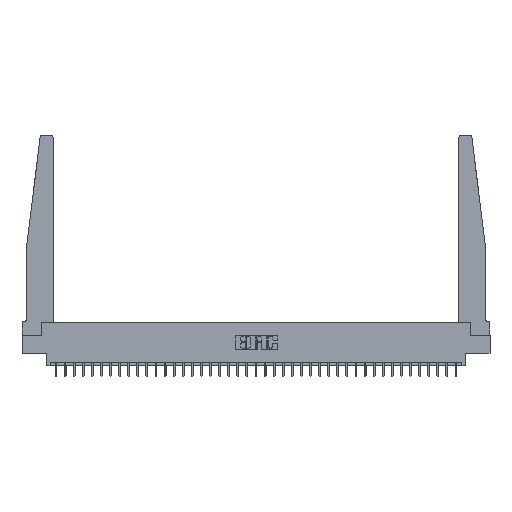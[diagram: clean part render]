
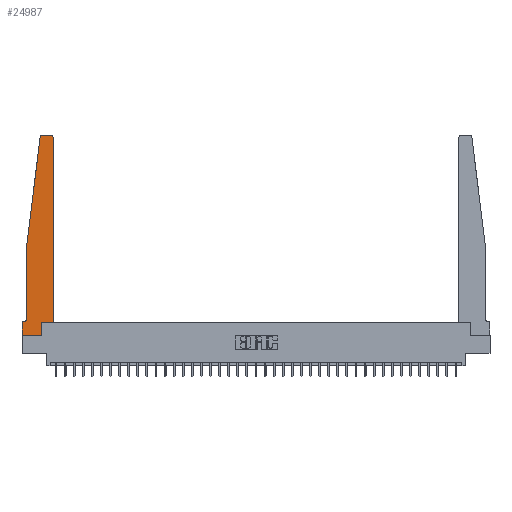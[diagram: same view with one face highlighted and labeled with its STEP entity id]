
A CAD part, top view. The second image highlights one B-rep face of the part: STEP entity #24987.
In plain terms, the highlighted planar face has unit normal (0, 0, 1).
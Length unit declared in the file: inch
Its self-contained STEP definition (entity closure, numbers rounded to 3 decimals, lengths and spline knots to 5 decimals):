
#27 = EDGE_CURVE ( 'NONE', #30497, #17124, #23463, .T. ) ;
#287 = CARTESIAN_POINT ( 'NONE',  ( 0., 0., 0.37 ) ) ;
#618 = AXIS2_PLACEMENT_3D ( 'NONE', #7165, #10270, #2116 ) ;
#1739 = DIRECTION ( 'NONE',  ( 1., 0., 0. ) ) ;
#2116 = DIRECTION ( 'NONE',  ( 1., 0., 0. ) ) ;
#2650 = VERTEX_POINT ( 'NONE', #287 ) ;
#3519 = CARTESIAN_POINT ( 'NONE',  ( 0.065, 0.1875, 0.37 ) ) ;
#5284 = VECTOR ( 'NONE', #30593, 39.37008 ) ;
#5538 = CARTESIAN_POINT ( 'NONE',  ( 0.425, 0.18, 0.37 ) ) ;
#5985 = CARTESIAN_POINT ( 'NONE',  ( 0.015, 0.1875, 0.37 ) ) ;
#6032 = CIRCLE ( 'NONE', #25410, 0.03 ) ;
#6417 = CIRCLE ( 'NONE', #11397, 0.05 ) ;
#7165 = CARTESIAN_POINT ( 'NONE',  ( 0., 0.1875, 0.37 ) ) ;
#7226 = VECTOR ( 'NONE', #32713, 39.37008 ) ;
#7527 = CARTESIAN_POINT ( 'NONE',  ( 0.2605, 0.18, 0.37 ) ) ;
#8022 = VERTEX_POINT ( 'NONE', #12897 ) ;
#8242 = AXIS2_PLACEMENT_3D ( 'NONE', #17707, #23071, #1739 ) ;
#8341 = EDGE_CURVE ( 'NONE', #2650, #33157, #9206, .T. ) ;
#8497 = VERTEX_POINT ( 'NONE', #12517 ) ;
#8962 = EDGE_CURVE ( 'NONE', #17124, #8022, #28455, .T. ) ;
#9074 = ORIENTED_EDGE ( 'NONE', *, *, #9526, .T. ) ;
#9206 = LINE ( 'NONE', #9385, #5284 ) ;
#9319 = EDGE_CURVE ( 'NONE', #31502, #16985, #12225, .T. ) ;
#9385 = CARTESIAN_POINT ( 'NONE',  ( 0., 0., 0.37 ) ) ;
#9450 = EDGE_CURVE ( 'NONE', #16985, #8497, #6032, .T. ) ;
#9526 = EDGE_CURVE ( 'NONE', #24720, #2650, #24337, .T. ) ;
#9711 = ORIENTED_EDGE ( 'NONE', *, *, #16611, .T. ) ;
#9835 = VERTEX_POINT ( 'NONE', #25703 ) ;
#10116 = CARTESIAN_POINT ( 'NONE',  ( 0.27653, 2.72, 0.37 ) ) ;
#10270 = DIRECTION ( 'NONE',  ( 0., 0., 1. ) ) ;
#11397 = AXIS2_PLACEMENT_3D ( 'NONE', #27478, #30103, #11688 ) ;
#11688 = DIRECTION ( 'NONE',  ( -1., 0., 0. ) ) ;
#12225 = LINE ( 'NONE', #22802, #24852 ) ;
#12517 = CARTESIAN_POINT ( 'NONE',  ( 0.24675, 2.72367, 0.37 ) ) ;
#12897 = CARTESIAN_POINT ( 'NONE',  ( 0.425, 2.72, 0.37 ) ) ;
#13628 = VECTOR ( 'NONE', #21528, 39.37008 ) ;
#14913 = CIRCLE ( 'NONE', #8242, 0.03 ) ;
#16009 = DIRECTION ( 'NONE',  ( 1., 0., 0. ) ) ;
#16269 = EDGE_CURVE ( 'NONE', #9835, #26635, #6417, .T. ) ;
#16300 = CARTESIAN_POINT ( 'NONE',  ( 0.065, 1.25, 0.37 ) ) ;
#16331 = LINE ( 'NONE', #21168, #13628 ) ;
#16611 = EDGE_CURVE ( 'NONE', #21790, #9835, #16331, .T. ) ;
#16985 = VERTEX_POINT ( 'NONE', #23419 ) ;
#17124 = VERTEX_POINT ( 'NONE', #5538 ) ;
#17304 = ORIENTED_EDGE ( 'NONE', *, *, #19566, .T. ) ;
#17484 = CARTESIAN_POINT ( 'NONE',  ( 0.065, 1.25, 0.37 ) ) ;
#17707 = CARTESIAN_POINT ( 'NONE',  ( 0.395, 2.72, 0.37 ) ) ;
#18349 = ORIENTED_EDGE ( 'NONE', *, *, #9319, .T. ) ;
#18661 = CARTESIAN_POINT ( 'NONE',  ( 0., 0.1875, 0.37 ) ) ;
#18758 = DIRECTION ( 'NONE',  ( 1., 0., 0. ) ) ;
#19566 = EDGE_CURVE ( 'NONE', #33157, #30497, #19835, .T. ) ;
#19835 = LINE ( 'NONE', #22263, #25959 ) ;
#20312 = EDGE_CURVE ( 'NONE', #8022, #31502, #14913, .T. ) ;
#20445 = CARTESIAN_POINT ( 'NONE',  ( 0.425, 0.18, 0.37 ) ) ;
#20695 = DIRECTION ( 'NONE',  ( 0., 0., 1. ) ) ;
#21054 = ORIENTED_EDGE ( 'NONE', *, *, #20312, .T. ) ;
#21168 = CARTESIAN_POINT ( 'NONE',  ( 0.065, 1.25, 0.37 ) ) ;
#21209 = ORIENTED_EDGE ( 'NONE', *, *, #9450, .T. ) ;
#21356 = CARTESIAN_POINT ( 'NONE',  ( 0.425, 0.18, 0.37 ) ) ;
#21528 = DIRECTION ( 'NONE',  ( 0., -1., 0. ) ) ;
#21547 = DIRECTION ( 'NONE',  ( 0., -1., 0. ) ) ;
#21790 = VERTEX_POINT ( 'NONE', #16300 ) ;
#22207 = VECTOR ( 'NONE', #28088, 39.37008 ) ;
#22263 = CARTESIAN_POINT ( 'NONE',  ( 0.2605, 0.18, 0.37 ) ) ;
#22347 = EDGE_LOOP ( 'NONE', ( #18349, #21209, #23995, #9711, #33280, #24533, #9074, #24364, #17304, #27841, #25458, #21054 ) ) ;
#22669 = VECTOR ( 'NONE', #21547, 39.37008 ) ;
#22802 = CARTESIAN_POINT ( 'NONE',  ( 0.25, 2.75, 0.37 ) ) ;
#23071 = DIRECTION ( 'NONE',  ( 0., 0., 1. ) ) ;
#23128 = DIRECTION ( 'NONE',  ( -1., 0., 0. ) ) ;
#23175 = VECTOR ( 'NONE', #23388, 39.37008 ) ;
#23294 = PLANE ( 'NONE',  #618 ) ;
#23388 = DIRECTION ( 'NONE',  ( 0., 1., 0. ) ) ;
#23419 = CARTESIAN_POINT ( 'NONE',  ( 0.27653, 2.75, 0.37 ) ) ;
#23463 = LINE ( 'NONE', #21356, #31782 ) ;
#23542 = EDGE_CURVE ( 'NONE', #26635, #24720, #27474, .T. ) ;
#23995 = ORIENTED_EDGE ( 'NONE', *, *, #30075, .T. ) ;
#24074 = CARTESIAN_POINT ( 'NONE',  ( 0.395, 2.75, 0.37 ) ) ;
#24337 = LINE ( 'NONE', #27451, #22669 ) ;
#24364 = ORIENTED_EDGE ( 'NONE', *, *, #8341, .T. ) ;
#24533 = ORIENTED_EDGE ( 'NONE', *, *, #23542, .T. ) ;
#24720 = VERTEX_POINT ( 'NONE', #18661 ) ;
#24852 = VECTOR ( 'NONE', #23128, 39.37008 ) ;
#24987 = ADVANCED_FACE ( 'NONE', ( #34242 ), #23294, .T. ) ;
#25286 = LINE ( 'NONE', #17484, #22207 ) ;
#25410 = AXIS2_PLACEMENT_3D ( 'NONE', #10116, #20695, #16009 ) ;
#25458 = ORIENTED_EDGE ( 'NONE', *, *, #8962, .T. ) ;
#25703 = CARTESIAN_POINT ( 'NONE',  ( 0.065, 0.2375, 0.37 ) ) ;
#25959 = VECTOR ( 'NONE', #30460, 39.37008 ) ;
#26635 = VERTEX_POINT ( 'NONE', #5985 ) ;
#27451 = CARTESIAN_POINT ( 'NONE',  ( 0., 0., 0.37 ) ) ;
#27474 = LINE ( 'NONE', #3519, #7226 ) ;
#27478 = CARTESIAN_POINT ( 'NONE',  ( 0.015, 0.2375, 0.37 ) ) ;
#27841 = ORIENTED_EDGE ( 'NONE', *, *, #27, .T. ) ;
#28088 = DIRECTION ( 'NONE',  ( -0.122, -0.992, 0. ) ) ;
#28455 = LINE ( 'NONE', #20445, #23175 ) ;
#28798 = CARTESIAN_POINT ( 'NONE',  ( 0.2605, 0., 0.37 ) ) ;
#30075 = EDGE_CURVE ( 'NONE', #8497, #21790, #25286, .T. ) ;
#30103 = DIRECTION ( 'NONE',  ( 0., 0., -1. ) ) ;
#30460 = DIRECTION ( 'NONE',  ( 0., 1., 0. ) ) ;
#30497 = VERTEX_POINT ( 'NONE', #7527 ) ;
#30593 = DIRECTION ( 'NONE',  ( 1., 0., 0. ) ) ;
#31502 = VERTEX_POINT ( 'NONE', #24074 ) ;
#31782 = VECTOR ( 'NONE', #18758, 39.37008 ) ;
#32713 = DIRECTION ( 'NONE',  ( -1., 0., 0. ) ) ;
#33157 = VERTEX_POINT ( 'NONE', #28798 ) ;
#33280 = ORIENTED_EDGE ( 'NONE', *, *, #16269, .T. ) ;
#34242 = FACE_OUTER_BOUND ( 'NONE', #22347, .T. ) ;
